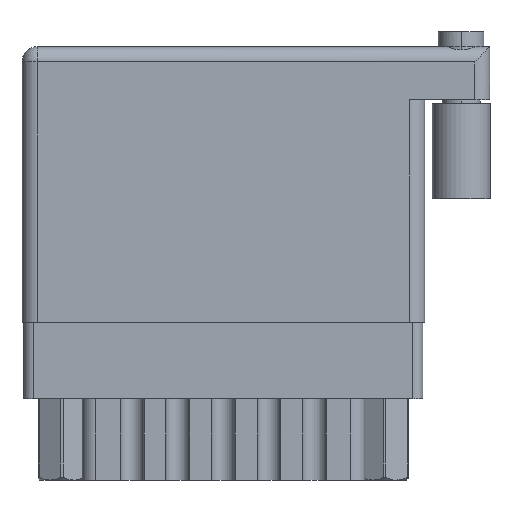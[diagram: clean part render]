
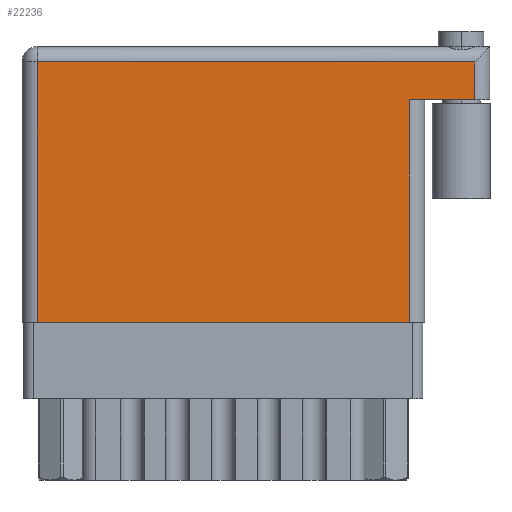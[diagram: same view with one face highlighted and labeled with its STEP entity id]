
A CAD part, front view. The second image highlights one B-rep face of the part: STEP entity #22236.
In plain terms, the highlighted face is planar.
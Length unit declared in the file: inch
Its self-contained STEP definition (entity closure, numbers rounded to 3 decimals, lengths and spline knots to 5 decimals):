
#389 = DIRECTION ( 'NONE',  ( -1., 0., 0. ) ) ;
#1038 = EDGE_CURVE ( 'NONE', #6848, #30546, #25469, .T. ) ;
#1322 = CARTESIAN_POINT ( 'NONE',  ( 0.05, 0., 0. ) ) ;
#1522 = EDGE_CURVE ( 'NONE', #25308, #6848, #27192, .T. ) ;
#1909 = VECTOR ( 'NONE', #24539, 39.37008 ) ;
#2239 = ORIENTED_EDGE ( 'NONE', *, *, #1522, .T. ) ;
#2525 = CARTESIAN_POINT ( 'NONE',  ( 1.539, 0.731, 0. ) ) ;
#2629 = DIRECTION ( 'NONE',  ( 0., 1., 0. ) ) ;
#5163 = LINE ( 'NONE', #2525, #30864 ) ;
#5966 = DIRECTION ( 'NONE',  ( 1., 0., 0. ) ) ;
#6848 = VERTEX_POINT ( 'NONE', #31844 ) ;
#7135 = VECTOR ( 'NONE', #33567, 39.37008 ) ;
#8145 = CARTESIAN_POINT ( 'NONE',  ( 0., 0., 0. ) ) ;
#9628 = EDGE_CURVE ( 'NONE', #30546, #10593, #27993, .T. ) ;
#10153 = VECTOR ( 'NONE', #5966, 39.37008 ) ;
#10227 = ORIENTED_EDGE ( 'NONE', *, *, #1038, .T. ) ;
#10305 = CARTESIAN_POINT ( 'NONE',  ( 1.489, 0.731, 0. ) ) ;
#10390 = ORIENTED_EDGE ( 'NONE', *, *, #9628, .T. ) ;
#10593 = VERTEX_POINT ( 'NONE', #18757 ) ;
#10606 = CARTESIAN_POINT ( 'NONE',  ( 0., 0.906, 0. ) ) ;
#11504 = ORIENTED_EDGE ( 'NONE', *, *, #20855, .T. ) ;
#12901 = FACE_OUTER_BOUND ( 'NONE', #32296, .T. ) ;
#13130 = EDGE_CURVE ( 'NONE', #21710, #24940, #5163, .T. ) ;
#13792 = CARTESIAN_POINT ( 'NONE',  ( 0., 0.856, 0. ) ) ;
#14623 = CARTESIAN_POINT ( 'NONE',  ( 1.489, 0.856, 0. ) ) ;
#15059 = VECTOR ( 'NONE', #34601, 39.37008 ) ;
#16266 = LINE ( 'NONE', #23840, #15059 ) ;
#18671 = LINE ( 'NONE', #29419, #29839 ) ;
#18757 = CARTESIAN_POINT ( 'NONE',  ( 1.275, 0., 0. ) ) ;
#20855 = EDGE_CURVE ( 'NONE', #10593, #24940, #18671, .T. ) ;
#21240 = CARTESIAN_POINT ( 'NONE',  ( 0.05, 0., 0. ) ) ;
#21531 = DIRECTION ( 'NONE',  ( -1., 0., 0. ) ) ;
#21710 = VERTEX_POINT ( 'NONE', #10305 ) ;
#22236 = ADVANCED_FACE ( 'NONE', ( #12901 ), #34753, .F. ) ;
#23840 = CARTESIAN_POINT ( 'NONE',  ( 1.489, 0.906, 0. ) ) ;
#24539 = DIRECTION ( 'NONE',  ( -1., 0., 0. ) ) ;
#24940 = VERTEX_POINT ( 'NONE', #29848 ) ;
#24997 = ORIENTED_EDGE ( 'NONE', *, *, #13130, .F. ) ;
#25308 = VERTEX_POINT ( 'NONE', #14623 ) ;
#25469 = LINE ( 'NONE', #1322, #7135 ) ;
#27192 = LINE ( 'NONE', #13792, #1909 ) ;
#27993 = LINE ( 'NONE', #8145, #10153 ) ;
#28807 = AXIS2_PLACEMENT_3D ( 'NONE', #10606, #29472, #21531 ) ;
#29419 = CARTESIAN_POINT ( 'NONE',  ( 1.275, 0.731, 0. ) ) ;
#29472 = DIRECTION ( 'NONE',  ( 0., 0., -1. ) ) ;
#29839 = VECTOR ( 'NONE', #2629, 39.37008 ) ;
#29848 = CARTESIAN_POINT ( 'NONE',  ( 1.275, 0.731, 0. ) ) ;
#30546 = VERTEX_POINT ( 'NONE', #21240 ) ;
#30864 = VECTOR ( 'NONE', #389, 39.37008 ) ;
#31844 = CARTESIAN_POINT ( 'NONE',  ( 0.05, 0.856, 0. ) ) ;
#32080 = ORIENTED_EDGE ( 'NONE', *, *, #32133, .T. ) ;
#32133 = EDGE_CURVE ( 'NONE', #21710, #25308, #16266, .T. ) ;
#32296 = EDGE_LOOP ( 'NONE', ( #10390, #11504, #24997, #32080, #2239, #10227 ) ) ;
#33567 = DIRECTION ( 'NONE',  ( 0., -1., 0. ) ) ;
#34601 = DIRECTION ( 'NONE',  ( 0., 1., 0. ) ) ;
#34753 = PLANE ( 'NONE',  #28807 ) ;
